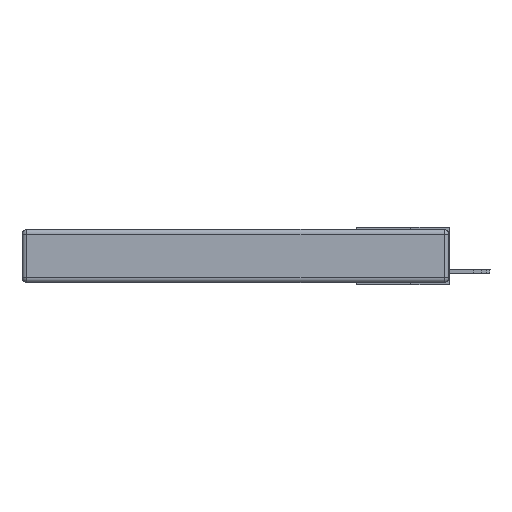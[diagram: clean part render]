
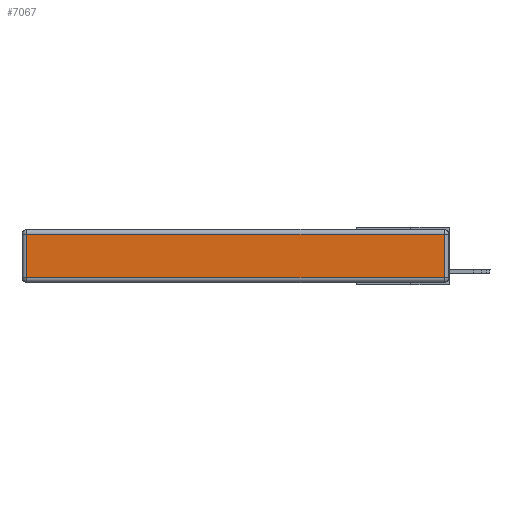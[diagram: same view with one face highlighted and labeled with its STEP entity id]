
A CAD part, left-side view. The second image highlights one B-rep face of the part: STEP entity #7067.
In plain terms, the highlighted planar face has unit normal (-1, 0, 0).
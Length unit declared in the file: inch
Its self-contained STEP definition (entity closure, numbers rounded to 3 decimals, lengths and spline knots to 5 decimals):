
#51 = VERTEX_POINT ( 'NONE', #11715 ) ;
#966 = AXIS2_PLACEMENT_3D ( 'NONE', #11947, #16270, #1636 ) ;
#1173 = VERTEX_POINT ( 'NONE', #6065 ) ;
#1636 = DIRECTION ( 'NONE',  ( 0., 0., 1. ) ) ;
#2068 = LINE ( 'NONE', #7806, #13175 ) ;
#2400 = DIRECTION ( 'NONE',  ( 0., -1., 0. ) ) ;
#3214 = LINE ( 'NONE', #15742, #12022 ) ;
#3698 = LINE ( 'NONE', #14168, #9277 ) ;
#4300 = PLANE ( 'NONE',  #966 ) ;
#5572 = ORIENTED_EDGE ( 'NONE', *, *, #12590, .T. ) ;
#6065 = CARTESIAN_POINT ( 'NONE',  ( 0., 2.72, -0.03 ) ) ;
#6339 = VECTOR ( 'NONE', #15052, 39.37008 ) ;
#6722 = ORIENTED_EDGE ( 'NONE', *, *, #11104, .T. ) ;
#7067 = ADVANCED_FACE ( 'NONE', ( #17941 ), #4300, .T. ) ;
#7474 = VERTEX_POINT ( 'NONE', #10371 ) ;
#7806 = CARTESIAN_POINT ( 'NONE',  ( 0., 2.72, -0.343 ) ) ;
#9277 = VECTOR ( 'NONE', #14040, 39.37008 ) ;
#9749 = CARTESIAN_POINT ( 'NONE',  ( 0., 2.72, -0.313 ) ) ;
#9976 = EDGE_CURVE ( 'NONE', #18004, #51, #3214, .T. ) ;
#10297 = LINE ( 'NONE', #14996, #6339 ) ;
#10371 = CARTESIAN_POINT ( 'NONE',  ( 0., 0.03, -0.03 ) ) ;
#10820 = ORIENTED_EDGE ( 'NONE', *, *, #13904, .T. ) ;
#11104 = EDGE_CURVE ( 'NONE', #51, #7474, #10297, .T. ) ;
#11715 = CARTESIAN_POINT ( 'NONE',  ( 0., 0.03, -0.313 ) ) ;
#11947 = CARTESIAN_POINT ( 'NONE',  ( 0., 0., -0.343 ) ) ;
#12022 = VECTOR ( 'NONE', #2400, 39.37008 ) ;
#12590 = EDGE_CURVE ( 'NONE', #7474, #1173, #3698, .T. ) ;
#13175 = VECTOR ( 'NONE', #16684, 39.37008 ) ;
#13904 = EDGE_CURVE ( 'NONE', #1173, #18004, #2068, .T. ) ;
#14040 = DIRECTION ( 'NONE',  ( 0., 1., 0. ) ) ;
#14168 = CARTESIAN_POINT ( 'NONE',  ( 0., 2.75, -0.03 ) ) ;
#14996 = CARTESIAN_POINT ( 'NONE',  ( 0., 0.03, -0.343 ) ) ;
#15052 = DIRECTION ( 'NONE',  ( 0., 0., 1. ) ) ;
#15145 = EDGE_LOOP ( 'NONE', ( #16737, #6722, #5572, #10820 ) ) ;
#15742 = CARTESIAN_POINT ( 'NONE',  ( 0., 0., -0.313 ) ) ;
#16270 = DIRECTION ( 'NONE',  ( -1., 0., 0. ) ) ;
#16684 = DIRECTION ( 'NONE',  ( 0., 0., -1. ) ) ;
#16737 = ORIENTED_EDGE ( 'NONE', *, *, #9976, .T. ) ;
#17941 = FACE_OUTER_BOUND ( 'NONE', #15145, .T. ) ;
#18004 = VERTEX_POINT ( 'NONE', #9749 ) ;
